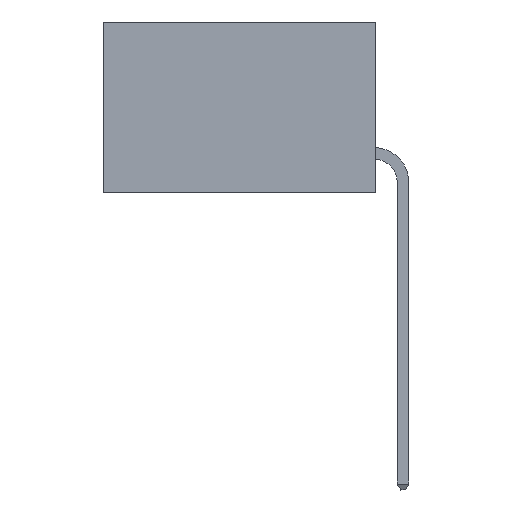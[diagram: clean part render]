
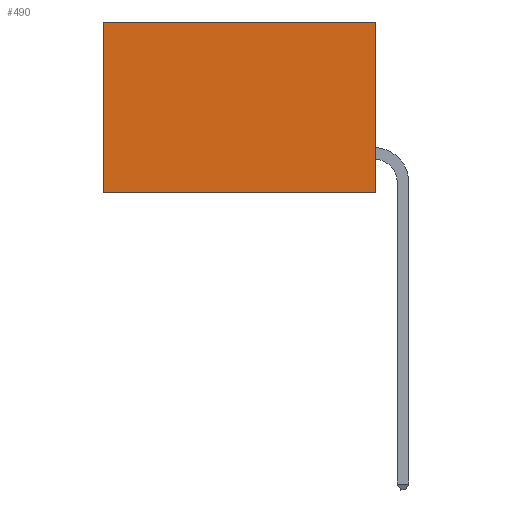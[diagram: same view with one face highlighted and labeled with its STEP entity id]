
A CAD part, left-side view. The second image highlights one B-rep face of the part: STEP entity #490.
In plain terms, the highlighted planar face has unit normal (-1, 0, 0).
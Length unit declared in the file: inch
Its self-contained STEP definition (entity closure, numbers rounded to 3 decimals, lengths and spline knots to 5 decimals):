
#184 = VECTOR ( 'NONE', #1340, 39.37008 ) ;
#490 = ADVANCED_FACE ( 'NONE', ( #14161 ), #14751, .F. ) ;
#1249 = VERTEX_POINT ( 'NONE', #2688 ) ;
#1340 = DIRECTION ( 'NONE',  ( 0., 0., -1. ) ) ;
#1413 = CARTESIAN_POINT ( 'NONE',  ( 0.277, 0., -0.37 ) ) ;
#1984 = EDGE_LOOP ( 'NONE', ( #12002, #11952, #6110, #5814 ) ) ;
#2451 = CARTESIAN_POINT ( 'NONE',  ( 0.277, 0., -0.37 ) ) ;
#2509 = EDGE_CURVE ( 'NONE', #2799, #1249, #13180, .T. ) ;
#2688 = CARTESIAN_POINT ( 'NONE',  ( 0.277, 0.59, -0.37 ) ) ;
#2799 = VERTEX_POINT ( 'NONE', #6119 ) ;
#5210 = EDGE_CURVE ( 'NONE', #13289, #18468, #16491, .T. ) ;
#5231 = CARTESIAN_POINT ( 'NONE',  ( 0.277, 0.59, -0.37 ) ) ;
#5814 = ORIENTED_EDGE ( 'NONE', *, *, #5210, .T. ) ;
#6110 = ORIENTED_EDGE ( 'NONE', *, *, #6724, .F. ) ;
#6119 = CARTESIAN_POINT ( 'NONE',  ( 0.277, 0., -0.37 ) ) ;
#6247 = CARTESIAN_POINT ( 'NONE',  ( 0.277, 0., 0. ) ) ;
#6709 = DIRECTION ( 'NONE',  ( 0., 0., -1. ) ) ;
#6724 = EDGE_CURVE ( 'NONE', #13289, #2799, #12148, .T. ) ;
#6904 = VECTOR ( 'NONE', #6709, 39.37008 ) ;
#7791 = DIRECTION ( 'NONE',  ( 1., 0., 0. ) ) ;
#7939 = DIRECTION ( 'NONE',  ( 0., 0., -1. ) ) ;
#8166 = VECTOR ( 'NONE', #18923, 39.37008 ) ;
#11377 = DIRECTION ( 'NONE',  ( 0., 1., 0. ) ) ;
#11952 = ORIENTED_EDGE ( 'NONE', *, *, #2509, .F. ) ;
#12002 = ORIENTED_EDGE ( 'NONE', *, *, #12286, .T. ) ;
#12148 = LINE ( 'NONE', #1413, #184 ) ;
#12286 = EDGE_CURVE ( 'NONE', #18468, #1249, #18550, .T. ) ;
#12718 = VECTOR ( 'NONE', #11377, 39.37008 ) ;
#13180 = LINE ( 'NONE', #2451, #12718 ) ;
#13289 = VERTEX_POINT ( 'NONE', #6247 ) ;
#14161 = FACE_OUTER_BOUND ( 'NONE', #1984, .T. ) ;
#14751 = PLANE ( 'NONE',  #16150 ) ;
#15556 = CARTESIAN_POINT ( 'NONE',  ( 0.277, 0., -0.37 ) ) ;
#16150 = AXIS2_PLACEMENT_3D ( 'NONE', #15556, #7791, #7939 ) ;
#16491 = LINE ( 'NONE', #18373, #8166 ) ;
#18373 = CARTESIAN_POINT ( 'NONE',  ( 0.277, 0., 0. ) ) ;
#18468 = VERTEX_POINT ( 'NONE', #19057 ) ;
#18550 = LINE ( 'NONE', #5231, #6904 ) ;
#18923 = DIRECTION ( 'NONE',  ( 0., 1., 0. ) ) ;
#19057 = CARTESIAN_POINT ( 'NONE',  ( 0.277, 0.59, 0. ) ) ;
